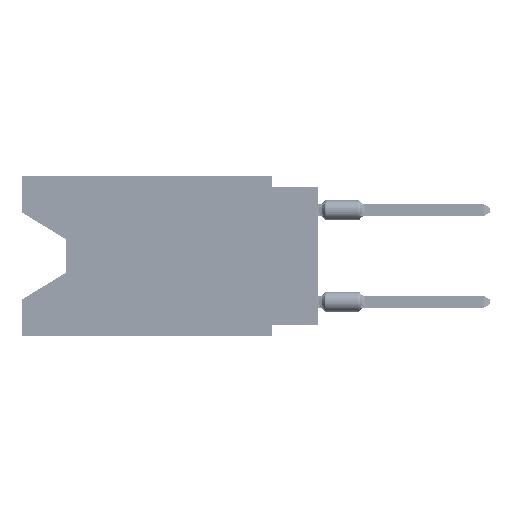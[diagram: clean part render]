
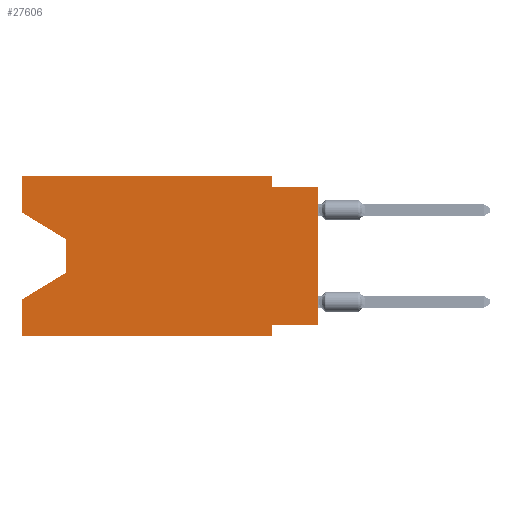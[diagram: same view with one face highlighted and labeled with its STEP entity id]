
A CAD part, left-side view. The second image highlights one B-rep face of the part: STEP entity #27606.
In plain terms, the highlighted planar face has unit normal (-1, 0, 0).
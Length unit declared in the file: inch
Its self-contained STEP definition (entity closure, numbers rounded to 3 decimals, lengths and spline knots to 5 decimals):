
#529 = DIRECTION ( 'NONE',  ( 0., 0., 1. ) ) ;
#2003 = VERTEX_POINT ( 'NONE', #17835 ) ;
#4108 = LINE ( 'NONE', #80006, #18754 ) ;
#4560 = DIRECTION ( 'NONE',  ( 0., 0., 1. ) ) ;
#5228 = DIRECTION ( 'NONE',  ( 0., -0.855, -0.519 ) ) ;
#6441 = PLANE ( 'NONE',  #26363 ) ;
#6602 = VERTEX_POINT ( 'NONE', #52993 ) ;
#6878 = VECTOR ( 'NONE', #13560, 39.37008 ) ;
#7300 = CARTESIAN_POINT ( 'NONE',  ( 0., 0.645, 0. ) ) ;
#9025 = LINE ( 'NONE', #30656, #18118 ) ;
#9113 = CARTESIAN_POINT ( 'NONE',  ( 0., 0.645, 0. ) ) ;
#9982 = CARTESIAN_POINT ( 'NONE',  ( 0., 0.1, -0.35 ) ) ;
#13185 = VECTOR ( 'NONE', #79107, 39.37008 ) ;
#13329 = EDGE_CURVE ( 'NONE', #20205, #16969, #9025, .T. ) ;
#13560 = DIRECTION ( 'NONE',  ( 0., 0., -1. ) ) ;
#14949 = VERTEX_POINT ( 'NONE', #16595 ) ;
#14973 = LINE ( 'NONE', #9982, #69804 ) ;
#15079 = CARTESIAN_POINT ( 'NONE',  ( 0., 0.55, -0.138 ) ) ;
#16595 = CARTESIAN_POINT ( 'NONE',  ( 0., 0., -0.325 ) ) ;
#16625 = VECTOR ( 'NONE', #86073, 39.37008 ) ;
#16969 = VERTEX_POINT ( 'NONE', #55819 ) ;
#17835 = CARTESIAN_POINT ( 'NONE',  ( 0., 0.645, -0.08025 ) ) ;
#18118 = VECTOR ( 'NONE', #71337, 39.37008 ) ;
#18177 = ORIENTED_EDGE ( 'NONE', *, *, #36211, .T. ) ;
#18754 = VECTOR ( 'NONE', #4560, 39.37008 ) ;
#19745 = CARTESIAN_POINT ( 'NONE',  ( 0., 0.645, -0.35 ) ) ;
#20205 = VERTEX_POINT ( 'NONE', #43605 ) ;
#20681 = ORIENTED_EDGE ( 'NONE', *, *, #34671, .F. ) ;
#23350 = EDGE_CURVE ( 'NONE', #28675, #20205, #54860, .T. ) ;
#24026 = LINE ( 'NONE', #51561, #38761 ) ;
#24576 = ORIENTED_EDGE ( 'NONE', *, *, #38395, .F. ) ;
#26363 = AXIS2_PLACEMENT_3D ( 'NONE', #89117, #39427, #53874 ) ;
#27606 = ADVANCED_FACE ( 'NONE', ( #40326 ), #6441, .F. ) ;
#28374 = EDGE_LOOP ( 'NONE', ( #40573, #38745, #47592, #24576, #18177, #78569, #54878, #69307, #68770, #20681, #61993, #62365 ) ) ;
#28675 = VERTEX_POINT ( 'NONE', #15079 ) ;
#29008 = EDGE_CURVE ( 'NONE', #6602, #33565, #14973, .T. ) ;
#29695 = CARTESIAN_POINT ( 'NONE',  ( 0., 0.645, -0.35 ) ) ;
#30656 = CARTESIAN_POINT ( 'NONE',  ( 0., 0.55, -0.212 ) ) ;
#32296 = DIRECTION ( 'NONE',  ( 0., 0., -1. ) ) ;
#32378 = EDGE_CURVE ( 'NONE', #75102, #76588, #51275, .T. ) ;
#33565 = VERTEX_POINT ( 'NONE', #72522 ) ;
#34671 = EDGE_CURVE ( 'NONE', #69777, #75102, #76323, .T. ) ;
#35012 = EDGE_CURVE ( 'NONE', #2003, #28675, #39540, .T. ) ;
#36211 = EDGE_CURVE ( 'NONE', #62169, #33565, #88846, .T. ) ;
#38395 = EDGE_CURVE ( 'NONE', #62169, #16969, #69173, .T. ) ;
#38734 = VECTOR ( 'NONE', #32296, 39.37008 ) ;
#38745 = ORIENTED_EDGE ( 'NONE', *, *, #23350, .T. ) ;
#38761 = VECTOR ( 'NONE', #79142, 39.37008 ) ;
#39427 = DIRECTION ( 'NONE',  ( 1., 0., 0. ) ) ;
#39540 = LINE ( 'NONE', #67546, #53031 ) ;
#40014 = CARTESIAN_POINT ( 'NONE',  ( 0., 0.1, 0. ) ) ;
#40326 = FACE_OUTER_BOUND ( 'NONE', #28374, .T. ) ;
#40573 = ORIENTED_EDGE ( 'NONE', *, *, #35012, .T. ) ;
#43605 = CARTESIAN_POINT ( 'NONE',  ( 0., 0.55, -0.212 ) ) ;
#43766 = LINE ( 'NONE', #64548, #82143 ) ;
#44064 = CARTESIAN_POINT ( 'NONE',  ( 0., 0., -0.025 ) ) ;
#47559 = EDGE_CURVE ( 'NONE', #69250, #69777, #72310, .T. ) ;
#47592 = ORIENTED_EDGE ( 'NONE', *, *, #13329, .T. ) ;
#48580 = DIRECTION ( 'NONE',  ( 0., -1., 0. ) ) ;
#51275 = LINE ( 'NONE', #44064, #16625 ) ;
#51561 = CARTESIAN_POINT ( 'NONE',  ( 0., 0., -0.325 ) ) ;
#52993 = CARTESIAN_POINT ( 'NONE',  ( 0., 0.1, -0.325 ) ) ;
#53031 = VECTOR ( 'NONE', #5228, 39.37008 ) ;
#53874 = DIRECTION ( 'NONE',  ( 0., 0., -1. ) ) ;
#54860 = LINE ( 'NONE', #82433, #38734 ) ;
#54878 = ORIENTED_EDGE ( 'NONE', *, *, #61349, .F. ) ;
#55819 = CARTESIAN_POINT ( 'NONE',  ( 0., 0.645, -0.26975 ) ) ;
#57509 = VECTOR ( 'NONE', #48580, 39.37008 ) ;
#61349 = EDGE_CURVE ( 'NONE', #14949, #6602, #24026, .T. ) ;
#61947 = VECTOR ( 'NONE', #529, 39.37008 ) ;
#61993 = ORIENTED_EDGE ( 'NONE', *, *, #47559, .F. ) ;
#62169 = VERTEX_POINT ( 'NONE', #29695 ) ;
#62365 = ORIENTED_EDGE ( 'NONE', *, *, #67836, .F. ) ;
#64548 = CARTESIAN_POINT ( 'NONE',  ( 0., 0.645, 0. ) ) ;
#67546 = CARTESIAN_POINT ( 'NONE',  ( 0., 0.645, -0.08025 ) ) ;
#67836 = EDGE_CURVE ( 'NONE', #2003, #69250, #43766, .T. ) ;
#68673 = CARTESIAN_POINT ( 'NONE',  ( 0., 0.1, -0.025 ) ) ;
#68735 = EDGE_CURVE ( 'NONE', #14949, #76588, #4108, .T. ) ;
#68770 = ORIENTED_EDGE ( 'NONE', *, *, #32378, .F. ) ;
#69173 = LINE ( 'NONE', #7300, #61947 ) ;
#69250 = VERTEX_POINT ( 'NONE', #72215 ) ;
#69307 = ORIENTED_EDGE ( 'NONE', *, *, #68735, .T. ) ;
#69777 = VERTEX_POINT ( 'NONE', #40014 ) ;
#69804 = VECTOR ( 'NONE', #83631, 39.37008 ) ;
#70431 = DIRECTION ( 'NONE',  ( 0., 0., 1. ) ) ;
#71337 = DIRECTION ( 'NONE',  ( 0., 0.855, -0.519 ) ) ;
#72215 = CARTESIAN_POINT ( 'NONE',  ( 0., 0.645, 0. ) ) ;
#72310 = LINE ( 'NONE', #9113, #13185 ) ;
#72522 = CARTESIAN_POINT ( 'NONE',  ( 0., 0.1, -0.35 ) ) ;
#75102 = VERTEX_POINT ( 'NONE', #68673 ) ;
#76323 = LINE ( 'NONE', #82222, #6878 ) ;
#76588 = VERTEX_POINT ( 'NONE', #83329 ) ;
#78569 = ORIENTED_EDGE ( 'NONE', *, *, #29008, .F. ) ;
#79107 = DIRECTION ( 'NONE',  ( 0., -1., 0. ) ) ;
#79142 = DIRECTION ( 'NONE',  ( 0., 1., 0. ) ) ;
#80006 = CARTESIAN_POINT ( 'NONE',  ( 0., 0., 0. ) ) ;
#82143 = VECTOR ( 'NONE', #70431, 39.37008 ) ;
#82222 = CARTESIAN_POINT ( 'NONE',  ( 0., 0.1, 0. ) ) ;
#82433 = CARTESIAN_POINT ( 'NONE',  ( 0., 0.55, -0.138 ) ) ;
#83329 = CARTESIAN_POINT ( 'NONE',  ( 0., 0., -0.025 ) ) ;
#83631 = DIRECTION ( 'NONE',  ( 0., 0., -1. ) ) ;
#86073 = DIRECTION ( 'NONE',  ( 0., -1., 0. ) ) ;
#88846 = LINE ( 'NONE', #19745, #57509 ) ;
#89117 = CARTESIAN_POINT ( 'NONE',  ( 0., 0.645, 0. ) ) ;
